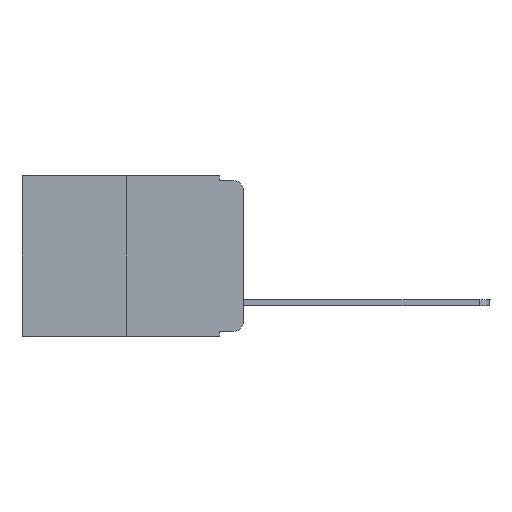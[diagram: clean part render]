
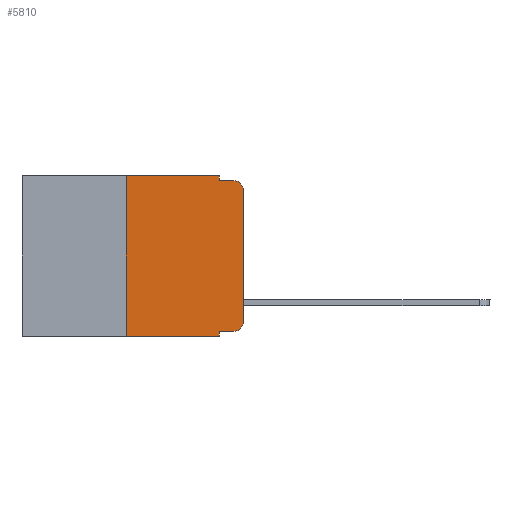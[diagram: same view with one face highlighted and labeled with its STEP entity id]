
A CAD part, left-side view. The second image highlights one B-rep face of the part: STEP entity #5810.
In plain terms, the highlighted planar face has unit normal (-1, 0, 0).
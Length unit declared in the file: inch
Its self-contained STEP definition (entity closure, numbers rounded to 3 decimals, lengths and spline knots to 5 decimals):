
#41 = VECTOR ( 'NONE', #4432, 39.37008 ) ;
#437 = VECTOR ( 'NONE', #9516, 39.37008 ) ;
#715 = DIRECTION ( 'NONE',  ( 0., 0., -1. ) ) ;
#774 = FACE_OUTER_BOUND ( 'NONE', #9648, .T. ) ;
#832 = CARTESIAN_POINT ( 'NONE',  ( 0., 0.473, 0. ) ) ;
#944 = CIRCLE ( 'NONE', #2330, 0.02 ) ;
#1148 = VECTOR ( 'NONE', #6619, 39.37008 ) ;
#1261 = DIRECTION ( 'NONE',  ( 0., 0., 1. ) ) ;
#1296 = DIRECTION ( 'NONE',  ( -1., 0., 0. ) ) ;
#1373 = ORIENTED_EDGE ( 'NONE', *, *, #4580, .F. ) ;
#1434 = CARTESIAN_POINT ( 'NONE',  ( 0., 0., -0.03 ) ) ;
#1495 = LINE ( 'NONE', #10638, #5154 ) ;
#1578 = ORIENTED_EDGE ( 'NONE', *, *, #4651, .T. ) ;
#1668 = VERTEX_POINT ( 'NONE', #4669 ) ;
#1757 = LINE ( 'NONE', #9925, #10273 ) ;
#1790 = EDGE_CURVE ( 'NONE', #5782, #5297, #4931, .T. ) ;
#1879 = ORIENTED_EDGE ( 'NONE', *, *, #5252, .T. ) ;
#1975 = CARTESIAN_POINT ( 'NONE',  ( 0., 0.02, -0.03 ) ) ;
#2330 = AXIS2_PLACEMENT_3D ( 'NONE', #1975, #2838, #10416 ) ;
#2376 = AXIS2_PLACEMENT_3D ( 'NONE', #832, #6761, #5938 ) ;
#2683 = CARTESIAN_POINT ( 'NONE',  ( 0., 0.051, -0.01 ) ) ;
#2696 = ORIENTED_EDGE ( 'NONE', *, *, #4062, .F. ) ;
#2717 = VECTOR ( 'NONE', #1261, 39.37008 ) ;
#2753 = CARTESIAN_POINT ( 'NONE',  ( 0., 0.051, -0.01 ) ) ;
#2838 = DIRECTION ( 'NONE',  ( -1., 0., 0. ) ) ;
#3145 = CARTESIAN_POINT ( 'NONE',  ( 0., 0.051, 0. ) ) ;
#3685 = CARTESIAN_POINT ( 'NONE',  ( 0., 0.02, -0.313 ) ) ;
#3799 = EDGE_CURVE ( 'NONE', #5297, #6750, #6179, .T. ) ;
#3896 = AXIS2_PLACEMENT_3D ( 'NONE', #3685, #1296, #9617 ) ;
#3897 = VERTEX_POINT ( 'NONE', #1434 ) ;
#3908 = VECTOR ( 'NONE', #5036, 39.37008 ) ;
#4062 = EDGE_CURVE ( 'NONE', #6077, #5782, #1757, .T. ) ;
#4080 = CARTESIAN_POINT ( 'NONE',  ( 0., 0.051, 0. ) ) ;
#4286 = ORIENTED_EDGE ( 'NONE', *, *, #3799, .F. ) ;
#4430 = ORIENTED_EDGE ( 'NONE', *, *, #7773, .T. ) ;
#4432 = DIRECTION ( 'NONE',  ( 0., -1., 0. ) ) ;
#4580 = EDGE_CURVE ( 'NONE', #5066, #6581, #7932, .T. ) ;
#4623 = LINE ( 'NONE', #8051, #2717 ) ;
#4651 = EDGE_CURVE ( 'NONE', #10738, #1668, #8598, .T. ) ;
#4669 = CARTESIAN_POINT ( 'NONE',  ( 0., 0., -0.313 ) ) ;
#4713 = VERTEX_POINT ( 'NONE', #10548 ) ;
#4867 = EDGE_CURVE ( 'NONE', #4713, #6077, #10050, .T. ) ;
#4931 = LINE ( 'NONE', #3145, #7429 ) ;
#5024 = DIRECTION ( 'NONE',  ( 0., -1., 0. ) ) ;
#5036 = DIRECTION ( 'NONE',  ( 0., 0., 1. ) ) ;
#5066 = VERTEX_POINT ( 'NONE', #7854 ) ;
#5154 = VECTOR ( 'NONE', #5024, 39.37008 ) ;
#5252 = EDGE_CURVE ( 'NONE', #5066, #10738, #1495, .T. ) ;
#5297 = VERTEX_POINT ( 'NONE', #2683 ) ;
#5322 = CARTESIAN_POINT ( 'NONE',  ( 0., 0.051, 0. ) ) ;
#5420 = CARTESIAN_POINT ( 'NONE',  ( 0., 0.02, -0.333 ) ) ;
#5782 = VERTEX_POINT ( 'NONE', #4080 ) ;
#5810 = ADVANCED_FACE ( 'NONE', ( #774 ), #9146, .F. ) ;
#5938 = DIRECTION ( 'NONE',  ( 0., 0., -1. ) ) ;
#6077 = VERTEX_POINT ( 'NONE', #6532 ) ;
#6179 = LINE ( 'NONE', #2753, #41 ) ;
#6532 = CARTESIAN_POINT ( 'NONE',  ( 0., 0.25, 0. ) ) ;
#6581 = VERTEX_POINT ( 'NONE', #10537 ) ;
#6619 = DIRECTION ( 'NONE',  ( 0., -1., 0. ) ) ;
#6750 = VERTEX_POINT ( 'NONE', #10086 ) ;
#6761 = DIRECTION ( 'NONE',  ( 1., 0., 0. ) ) ;
#6792 = EDGE_CURVE ( 'NONE', #3897, #6750, #944, .T. ) ;
#7429 = VECTOR ( 'NONE', #715, 39.37008 ) ;
#7435 = CARTESIAN_POINT ( 'NONE',  ( 0., 0.473, -0.343 ) ) ;
#7703 = CARTESIAN_POINT ( 'NONE',  ( 0., 0.25, 0. ) ) ;
#7773 = EDGE_CURVE ( 'NONE', #4713, #6581, #9166, .T. ) ;
#7854 = CARTESIAN_POINT ( 'NONE',  ( 0., 0.051, -0.333 ) ) ;
#7932 = LINE ( 'NONE', #5322, #437 ) ;
#8051 = CARTESIAN_POINT ( 'NONE',  ( 0., 0., 0. ) ) ;
#8437 = ORIENTED_EDGE ( 'NONE', *, *, #8585, .T. ) ;
#8585 = EDGE_CURVE ( 'NONE', #1668, #3897, #4623, .T. ) ;
#8598 = CIRCLE ( 'NONE', #3896, 0.02 ) ;
#9146 = PLANE ( 'NONE',  #2376 ) ;
#9166 = LINE ( 'NONE', #7435, #1148 ) ;
#9256 = ORIENTED_EDGE ( 'NONE', *, *, #4867, .F. ) ;
#9407 = ORIENTED_EDGE ( 'NONE', *, *, #6792, .T. ) ;
#9516 = DIRECTION ( 'NONE',  ( 0., 0., -1. ) ) ;
#9617 = DIRECTION ( 'NONE',  ( 0., 0., -1. ) ) ;
#9648 = EDGE_LOOP ( 'NONE', ( #8437, #9407, #4286, #10125, #2696, #9256, #4430, #1373, #1879, #1578 ) ) ;
#9925 = CARTESIAN_POINT ( 'NONE',  ( 0., 0.473, 0. ) ) ;
#9975 = DIRECTION ( 'NONE',  ( 0., -1., 0. ) ) ;
#10050 = LINE ( 'NONE', #7703, #3908 ) ;
#10086 = CARTESIAN_POINT ( 'NONE',  ( 0., 0.02, -0.01 ) ) ;
#10125 = ORIENTED_EDGE ( 'NONE', *, *, #1790, .F. ) ;
#10273 = VECTOR ( 'NONE', #9975, 39.37008 ) ;
#10416 = DIRECTION ( 'NONE',  ( 0., 0., -1. ) ) ;
#10537 = CARTESIAN_POINT ( 'NONE',  ( 0., 0.051, -0.343 ) ) ;
#10548 = CARTESIAN_POINT ( 'NONE',  ( 0., 0.25, -0.343 ) ) ;
#10638 = CARTESIAN_POINT ( 'NONE',  ( 0., 0.051, -0.333 ) ) ;
#10738 = VERTEX_POINT ( 'NONE', #5420 ) ;
